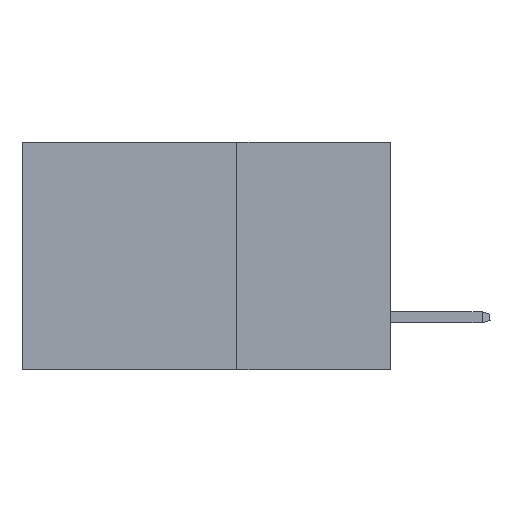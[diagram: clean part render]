
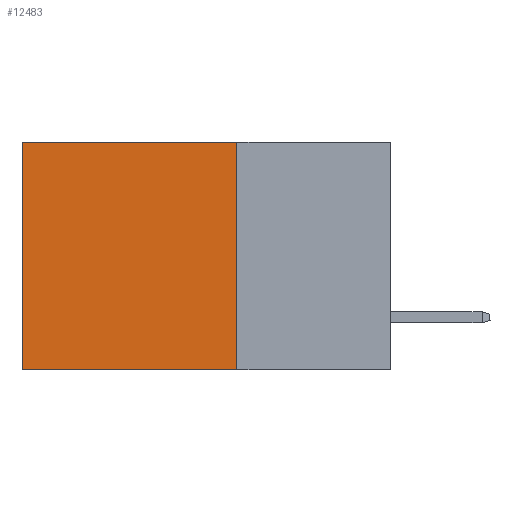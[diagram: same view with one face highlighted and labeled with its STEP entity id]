
A CAD part, left-side view. The second image highlights one B-rep face of the part: STEP entity #12483.
In plain terms, the highlighted planar face has unit normal (-1, 0, 0).
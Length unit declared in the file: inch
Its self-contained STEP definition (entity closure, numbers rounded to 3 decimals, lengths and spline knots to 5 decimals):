
#18 = VECTOR ( 'NONE', #5832, 39.37008 ) ;
#140 = CARTESIAN_POINT ( 'NONE',  ( 0.2875, 0.25, 0. ) ) ;
#463 = VERTEX_POINT ( 'NONE', #814 ) ;
#611 = VERTEX_POINT ( 'NONE', #2600 ) ;
#687 = ORIENTED_EDGE ( 'NONE', *, *, #10825, .F. ) ;
#814 = CARTESIAN_POINT ( 'NONE',  ( 0.2875, 0.6, 0. ) ) ;
#1142 = FACE_OUTER_BOUND ( 'NONE', #7684, .T. ) ;
#1298 = AXIS2_PLACEMENT_3D ( 'NONE', #1506, #9527, #4498 ) ;
#1506 = CARTESIAN_POINT ( 'NONE',  ( 0.2875, 0.25, 0. ) ) ;
#1917 = CARTESIAN_POINT ( 'NONE',  ( 0.2875, 0.25, 0. ) ) ;
#2084 = LINE ( 'NONE', #3146, #9187 ) ;
#2196 = PLANE ( 'NONE',  #1298 ) ;
#2600 = CARTESIAN_POINT ( 'NONE',  ( 0.2875, 0.6, -0.37 ) ) ;
#2937 = VECTOR ( 'NONE', #11817, 39.37008 ) ;
#3146 = CARTESIAN_POINT ( 'NONE',  ( 0.2875, 0.6, 0. ) ) ;
#3252 = LINE ( 'NONE', #4689, #2937 ) ;
#4037 = DIRECTION ( 'NONE',  ( 0., 1., 0. ) ) ;
#4498 = DIRECTION ( 'NONE',  ( 0., 0., -1. ) ) ;
#4689 = CARTESIAN_POINT ( 'NONE',  ( 0.2875, 0.25, 0. ) ) ;
#5141 = EDGE_CURVE ( 'NONE', #6915, #611, #5618, .T. ) ;
#5618 = LINE ( 'NONE', #10123, #10377 ) ;
#5625 = ORIENTED_EDGE ( 'NONE', *, *, #5141, .F. ) ;
#5832 = DIRECTION ( 'NONE',  ( 0., 1., 0. ) ) ;
#6634 = VERTEX_POINT ( 'NONE', #140 ) ;
#6811 = ORIENTED_EDGE ( 'NONE', *, *, #6974, .T. ) ;
#6915 = VERTEX_POINT ( 'NONE', #7701 ) ;
#6974 = EDGE_CURVE ( 'NONE', #6634, #463, #12367, .T. ) ;
#7684 = EDGE_LOOP ( 'NONE', ( #8827, #5625, #687, #6811 ) ) ;
#7701 = CARTESIAN_POINT ( 'NONE',  ( 0.2875, 0.25, -0.37 ) ) ;
#7812 = EDGE_CURVE ( 'NONE', #463, #611, #2084, .T. ) ;
#8217 = DIRECTION ( 'NONE',  ( 0., 0., -1. ) ) ;
#8827 = ORIENTED_EDGE ( 'NONE', *, *, #7812, .T. ) ;
#9187 = VECTOR ( 'NONE', #8217, 39.37008 ) ;
#9527 = DIRECTION ( 'NONE',  ( 1., 0., 0. ) ) ;
#10123 = CARTESIAN_POINT ( 'NONE',  ( 0.2875, 0.25, -0.37 ) ) ;
#10377 = VECTOR ( 'NONE', #4037, 39.37008 ) ;
#10825 = EDGE_CURVE ( 'NONE', #6634, #6915, #3252, .T. ) ;
#11817 = DIRECTION ( 'NONE',  ( 0., 0., -1. ) ) ;
#12367 = LINE ( 'NONE', #1917, #18 ) ;
#12483 = ADVANCED_FACE ( 'NONE', ( #1142 ), #2196, .F. ) ;
